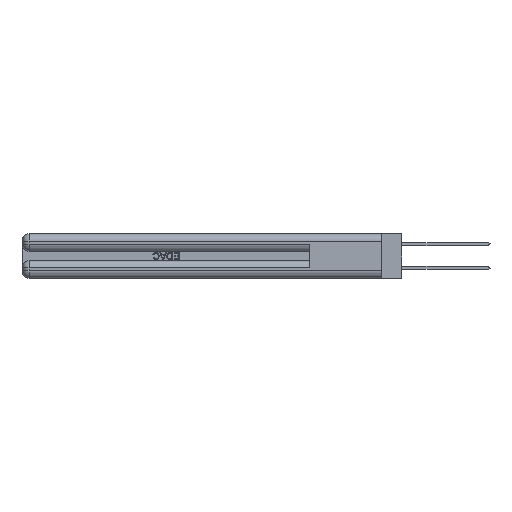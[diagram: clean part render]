
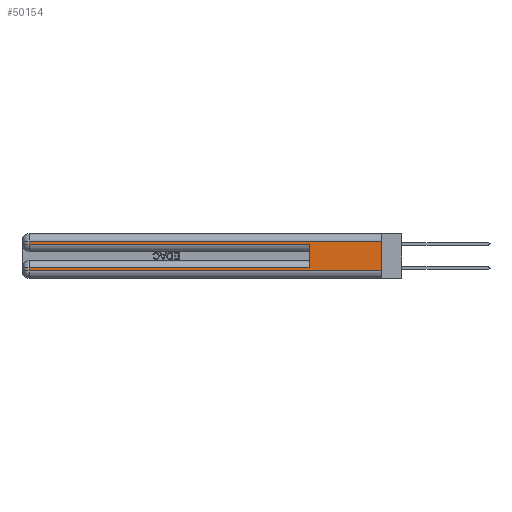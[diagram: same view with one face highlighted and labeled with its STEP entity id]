
A CAD part, left-side view. The second image highlights one B-rep face of the part: STEP entity #50154.
In plain terms, the highlighted planar face has unit normal (-1, 0, 0).
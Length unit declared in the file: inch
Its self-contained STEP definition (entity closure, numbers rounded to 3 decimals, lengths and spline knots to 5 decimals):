
#195 = VERTEX_POINT ( 'NONE', #41141 ) ;
#729 = VECTOR ( 'NONE', #13151, 39.37008 ) ;
#968 = CARTESIAN_POINT ( 'NONE',  ( 0., 2.94, 0.37 ) ) ;
#1157 = ORIENTED_EDGE ( 'NONE', *, *, #26773, .T. ) ;
#1905 = DIRECTION ( 'NONE',  ( 0., 1., 0. ) ) ;
#2479 = VERTEX_POINT ( 'NONE', #49931 ) ;
#2751 = CARTESIAN_POINT ( 'NONE',  ( 0., 0.6, 0.085 ) ) ;
#3405 = DIRECTION ( 'NONE',  ( 1., 0., 0. ) ) ;
#4254 = CARTESIAN_POINT ( 'NONE',  ( 0., 2.94, 0.085 ) ) ;
#4988 = DIRECTION ( 'NONE',  ( 0., 0., -1. ) ) ;
#5319 = EDGE_CURVE ( 'NONE', #2479, #12026, #6510, .T. ) ;
#5528 = LINE ( 'NONE', #45929, #25613 ) ;
#5763 = CARTESIAN_POINT ( 'NONE',  ( 0., 0., 0.085 ) ) ;
#6361 = EDGE_CURVE ( 'NONE', #27925, #195, #33370, .T. ) ;
#6510 = LINE ( 'NONE', #18995, #47889 ) ;
#6571 = CARTESIAN_POINT ( 'NONE',  ( 0., 0., 0.31 ) ) ;
#7592 = CARTESIAN_POINT ( 'NONE',  ( 0., 0., 0.37 ) ) ;
#8499 = LINE ( 'NONE', #7592, #48620 ) ;
#8585 = CARTESIAN_POINT ( 'NONE',  ( 0., 2.94, 0.285 ) ) ;
#9328 = LINE ( 'NONE', #29628, #37667 ) ;
#10781 = VECTOR ( 'NONE', #4988, 39.37008 ) ;
#12026 = VERTEX_POINT ( 'NONE', #8585 ) ;
#13151 = DIRECTION ( 'NONE',  ( 0., -1., 0. ) ) ;
#15410 = VECTOR ( 'NONE', #25934, 39.37008 ) ;
#15414 = DIRECTION ( 'NONE',  ( 0., 0., 1. ) ) ;
#18396 = CARTESIAN_POINT ( 'NONE',  ( 0., 0.6, 0.285 ) ) ;
#18705 = ORIENTED_EDGE ( 'NONE', *, *, #33010, .F. ) ;
#18995 = CARTESIAN_POINT ( 'NONE',  ( 0., 2.94, 0.37 ) ) ;
#19017 = VERTEX_POINT ( 'NONE', #6571 ) ;
#19373 = CARTESIAN_POINT ( 'NONE',  ( 0., 0., 0.37 ) ) ;
#21477 = VERTEX_POINT ( 'NONE', #27875 ) ;
#22518 = ORIENTED_EDGE ( 'NONE', *, *, #49552, .F. ) ;
#24811 = LINE ( 'NONE', #5763, #15410 ) ;
#25613 = VECTOR ( 'NONE', #1905, 39.37008 ) ;
#25934 = DIRECTION ( 'NONE',  ( 0., 1., 0. ) ) ;
#26036 = AXIS2_PLACEMENT_3D ( 'NONE', #19373, #3405, #31480 ) ;
#26773 = EDGE_CURVE ( 'NONE', #12026, #37211, #42171, .T. ) ;
#27078 = DIRECTION ( 'NONE',  ( 0., 0., -1. ) ) ;
#27255 = LINE ( 'NONE', #39451, #36666 ) ;
#27875 = CARTESIAN_POINT ( 'NONE',  ( 0., 0., 0.06 ) ) ;
#27925 = VERTEX_POINT ( 'NONE', #4254 ) ;
#28917 = EDGE_CURVE ( 'NONE', #19017, #2479, #5528, .T. ) ;
#29628 = CARTESIAN_POINT ( 'NONE',  ( 0., 0., 0.06 ) ) ;
#31228 = EDGE_CURVE ( 'NONE', #35922, #27925, #24811, .T. ) ;
#31306 = PLANE ( 'NONE',  #26036 ) ;
#31480 = DIRECTION ( 'NONE',  ( 0., 0., -1. ) ) ;
#31913 = ORIENTED_EDGE ( 'NONE', *, *, #5319, .T. ) ;
#33010 = EDGE_CURVE ( 'NONE', #19017, #21477, #8499, .T. ) ;
#33138 = CARTESIAN_POINT ( 'NONE',  ( 0., 0., 0.285 ) ) ;
#33370 = LINE ( 'NONE', #968, #10781 ) ;
#33685 = DIRECTION ( 'NONE',  ( 0., -1., 0. ) ) ;
#34283 = EDGE_LOOP ( 'NONE', ( #18705, #40071, #31913, #1157, #22518, #35710, #46354, #39468 ) ) ;
#35710 = ORIENTED_EDGE ( 'NONE', *, *, #31228, .T. ) ;
#35922 = VERTEX_POINT ( 'NONE', #2751 ) ;
#36666 = VECTOR ( 'NONE', #15414, 39.37008 ) ;
#37211 = VERTEX_POINT ( 'NONE', #18396 ) ;
#37667 = VECTOR ( 'NONE', #33685, 39.37008 ) ;
#39451 = CARTESIAN_POINT ( 'NONE',  ( 0., 0.6, 0.145 ) ) ;
#39468 = ORIENTED_EDGE ( 'NONE', *, *, #47281, .T. ) ;
#40071 = ORIENTED_EDGE ( 'NONE', *, *, #28917, .T. ) ;
#41141 = CARTESIAN_POINT ( 'NONE',  ( 0., 2.94, 0.06 ) ) ;
#42171 = LINE ( 'NONE', #33138, #729 ) ;
#45929 = CARTESIAN_POINT ( 'NONE',  ( 0., 0., 0.31 ) ) ;
#46354 = ORIENTED_EDGE ( 'NONE', *, *, #6361, .T. ) ;
#47281 = EDGE_CURVE ( 'NONE', #195, #21477, #9328, .T. ) ;
#47562 = DIRECTION ( 'NONE',  ( 0., 0., -1. ) ) ;
#47889 = VECTOR ( 'NONE', #27078, 39.37008 ) ;
#48620 = VECTOR ( 'NONE', #47562, 39.37008 ) ;
#49552 = EDGE_CURVE ( 'NONE', #35922, #37211, #27255, .T. ) ;
#49931 = CARTESIAN_POINT ( 'NONE',  ( 0., 2.94, 0.31 ) ) ;
#50154 = ADVANCED_FACE ( 'NONE', ( #51101 ), #31306, .F. ) ;
#51101 = FACE_OUTER_BOUND ( 'NONE', #34283, .T. ) ;
